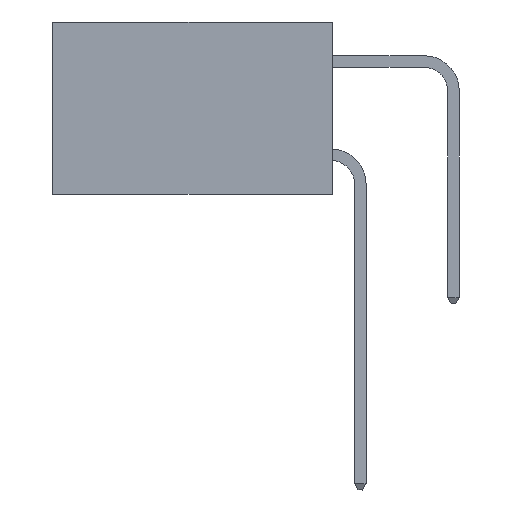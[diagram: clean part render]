
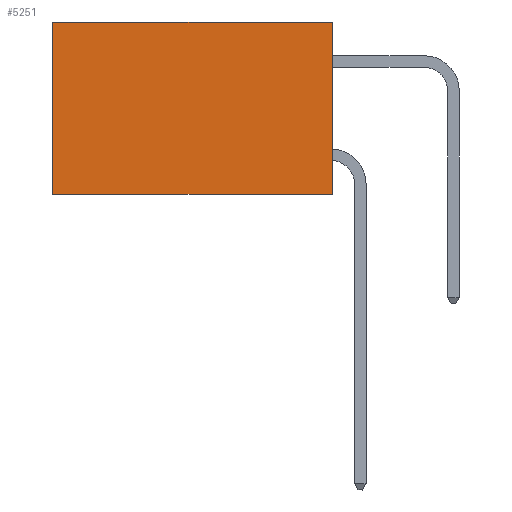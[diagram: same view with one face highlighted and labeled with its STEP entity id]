
A CAD part, left-side view. The second image highlights one B-rep face of the part: STEP entity #5251.
In plain terms, the highlighted planar face has unit normal (-1, 0, 0).
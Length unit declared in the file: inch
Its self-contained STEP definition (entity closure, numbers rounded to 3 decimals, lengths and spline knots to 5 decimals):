
#201 = ORIENTED_EDGE ( 'NONE', *, *, #4261, .F. ) ;
#443 = DIRECTION ( 'NONE',  ( 0., 0., -1. ) ) ;
#567 = CARTESIAN_POINT ( 'NONE',  ( 0.2615, 0., 0. ) ) ;
#1543 = ORIENTED_EDGE ( 'NONE', *, *, #3832, .T. ) ;
#1944 = CARTESIAN_POINT ( 'NONE',  ( 0.2615, 0., -0.37 ) ) ;
#2297 = VERTEX_POINT ( 'NONE', #11034 ) ;
#2636 = ORIENTED_EDGE ( 'NONE', *, *, #3487, .F. ) ;
#2888 = VERTEX_POINT ( 'NONE', #4381 ) ;
#2909 = LINE ( 'NONE', #10806, #4631 ) ;
#2958 = DIRECTION ( 'NONE',  ( 0., 0., -1. ) ) ;
#3411 = LINE ( 'NONE', #4084, #9276 ) ;
#3487 = EDGE_CURVE ( 'NONE', #2888, #5092, #3411, .T. ) ;
#3832 = EDGE_CURVE ( 'NONE', #4251, #5092, #2909, .T. ) ;
#3912 = CARTESIAN_POINT ( 'NONE',  ( 0.2615, 0., -0.37 ) ) ;
#4037 = VECTOR ( 'NONE', #4756, 39.37008 ) ;
#4084 = CARTESIAN_POINT ( 'NONE',  ( 0.2615, 0., -0.37 ) ) ;
#4251 = VERTEX_POINT ( 'NONE', #9623 ) ;
#4261 = EDGE_CURVE ( 'NONE', #2297, #2888, #7024, .T. ) ;
#4381 = CARTESIAN_POINT ( 'NONE',  ( 0.2615, 0., -0.37 ) ) ;
#4457 = ORIENTED_EDGE ( 'NONE', *, *, #5701, .T. ) ;
#4631 = VECTOR ( 'NONE', #443, 39.37008 ) ;
#4748 = PLANE ( 'NONE',  #10594 ) ;
#4756 = DIRECTION ( 'NONE',  ( 0., 1., 0. ) ) ;
#4865 = FACE_OUTER_BOUND ( 'NONE', #9829, .T. ) ;
#5092 = VERTEX_POINT ( 'NONE', #6204 ) ;
#5251 = ADVANCED_FACE ( 'NONE', ( #4865 ), #4748, .F. ) ;
#5701 = EDGE_CURVE ( 'NONE', #2297, #4251, #10588, .T. ) ;
#6204 = CARTESIAN_POINT ( 'NONE',  ( 0.2615, 0.6, -0.37 ) ) ;
#7024 = LINE ( 'NONE', #1944, #10250 ) ;
#8767 = DIRECTION ( 'NONE',  ( 0., 0., -1. ) ) ;
#9239 = DIRECTION ( 'NONE',  ( 0., 1., 0. ) ) ;
#9276 = VECTOR ( 'NONE', #9239, 39.37008 ) ;
#9623 = CARTESIAN_POINT ( 'NONE',  ( 0.2615, 0.6, 0. ) ) ;
#9829 = EDGE_LOOP ( 'NONE', ( #1543, #2636, #201, #4457 ) ) ;
#10250 = VECTOR ( 'NONE', #8767, 39.37008 ) ;
#10588 = LINE ( 'NONE', #567, #4037 ) ;
#10594 = AXIS2_PLACEMENT_3D ( 'NONE', #3912, #10633, #2958 ) ;
#10633 = DIRECTION ( 'NONE',  ( 1., 0., 0. ) ) ;
#10806 = CARTESIAN_POINT ( 'NONE',  ( 0.2615, 0.6, -0.37 ) ) ;
#11034 = CARTESIAN_POINT ( 'NONE',  ( 0.2615, 0., 0. ) ) ;
